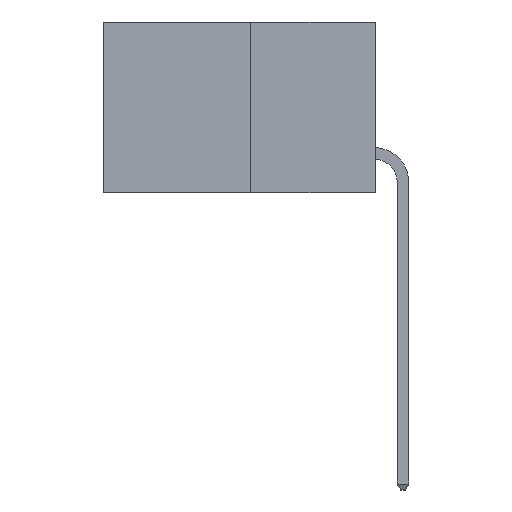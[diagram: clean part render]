
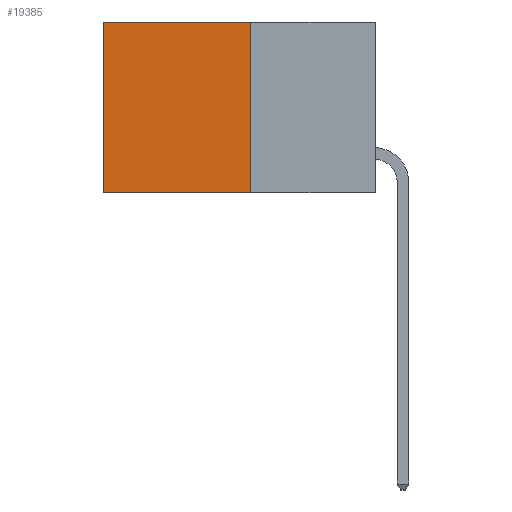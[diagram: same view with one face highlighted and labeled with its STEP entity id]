
A CAD part, left-side view. The second image highlights one B-rep face of the part: STEP entity #19385.
In plain terms, the highlighted planar face has unit normal (-1, 0, 0).
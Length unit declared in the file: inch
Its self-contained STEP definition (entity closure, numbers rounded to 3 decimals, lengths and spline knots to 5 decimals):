
#1745 = VERTEX_POINT ( 'NONE', #14704 ) ;
#2129 = DIRECTION ( 'NONE',  ( 0., 0., -1. ) ) ;
#2132 = VECTOR ( 'NONE', #16103, 39.37008 ) ;
#2828 = LINE ( 'NONE', #16594, #2132 ) ;
#3560 = CARTESIAN_POINT ( 'NONE',  ( 0.277, 0.27, 0. ) ) ;
#3714 = CARTESIAN_POINT ( 'NONE',  ( 0.277, 0.59, -0.37 ) ) ;
#4312 = EDGE_CURVE ( 'NONE', #7407, #14297, #2828, .T. ) ;
#4652 = EDGE_CURVE ( 'NONE', #25766, #1745, #10741, .T. ) ;
#5511 = CARTESIAN_POINT ( 'NONE',  ( 0.277, 0.59, 0. ) ) ;
#6692 = VECTOR ( 'NONE', #12018, 39.37008 ) ;
#7407 = VERTEX_POINT ( 'NONE', #5511 ) ;
#7463 = EDGE_LOOP ( 'NONE', ( #26328, #13993, #17867, #11613 ) ) ;
#9689 = DIRECTION ( 'NONE',  ( 0., 0., -1. ) ) ;
#10060 = CARTESIAN_POINT ( 'NONE',  ( 0.277, 0.27, -0.37 ) ) ;
#10552 = LINE ( 'NONE', #3560, #21132 ) ;
#10741 = LINE ( 'NONE', #10060, #15868 ) ;
#11613 = ORIENTED_EDGE ( 'NONE', *, *, #17334, .T. ) ;
#12018 = DIRECTION ( 'NONE',  ( 0., 1., 0. ) ) ;
#12356 = EDGE_CURVE ( 'NONE', #1745, #14297, #12550, .T. ) ;
#12550 = LINE ( 'NONE', #22802, #6692 ) ;
#13111 = CARTESIAN_POINT ( 'NONE',  ( 0.277, 0.27, -0.37 ) ) ;
#13993 = ORIENTED_EDGE ( 'NONE', *, *, #12356, .F. ) ;
#14297 = VERTEX_POINT ( 'NONE', #3714 ) ;
#14704 = CARTESIAN_POINT ( 'NONE',  ( 0.277, 0.27, -0.37 ) ) ;
#15294 = DIRECTION ( 'NONE',  ( 1., 0., 0. ) ) ;
#15868 = VECTOR ( 'NONE', #9689, 39.37008 ) ;
#16103 = DIRECTION ( 'NONE',  ( 0., 0., -1. ) ) ;
#16594 = CARTESIAN_POINT ( 'NONE',  ( 0.277, 0.59, -0.37 ) ) ;
#17334 = EDGE_CURVE ( 'NONE', #25766, #7407, #10552, .T. ) ;
#17867 = ORIENTED_EDGE ( 'NONE', *, *, #4652, .F. ) ;
#19385 = ADVANCED_FACE ( 'NONE', ( #26853 ), #26031, .F. ) ;
#21132 = VECTOR ( 'NONE', #27510, 39.37008 ) ;
#22802 = CARTESIAN_POINT ( 'NONE',  ( 0.277, 0.27, -0.37 ) ) ;
#23959 = CARTESIAN_POINT ( 'NONE',  ( 0.277, 0.27, 0. ) ) ;
#24787 = AXIS2_PLACEMENT_3D ( 'NONE', #13111, #15294, #2129 ) ;
#25766 = VERTEX_POINT ( 'NONE', #23959 ) ;
#26031 = PLANE ( 'NONE',  #24787 ) ;
#26328 = ORIENTED_EDGE ( 'NONE', *, *, #4312, .T. ) ;
#26853 = FACE_OUTER_BOUND ( 'NONE', #7463, .T. ) ;
#27510 = DIRECTION ( 'NONE',  ( 0., 1., 0. ) ) ;
